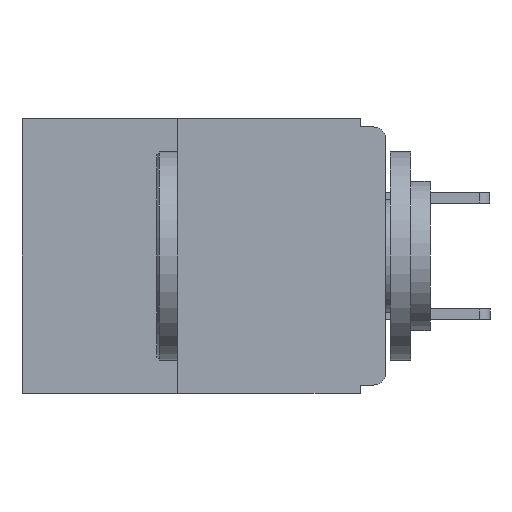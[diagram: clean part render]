
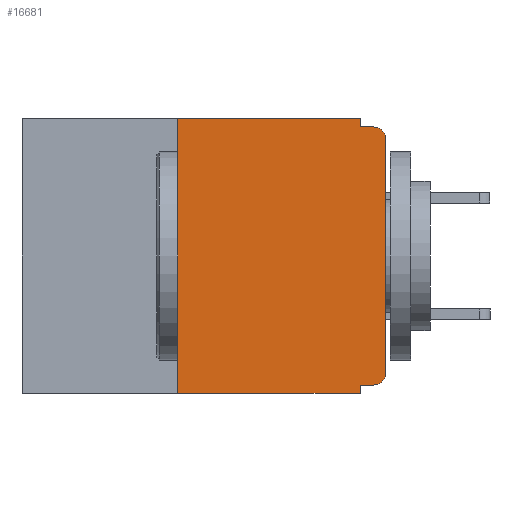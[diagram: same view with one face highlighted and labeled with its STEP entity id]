
A CAD part, left-side view. The second image highlights one B-rep face of the part: STEP entity #16681.
In plain terms, the highlighted planar face has unit normal (-1, 0, 0).
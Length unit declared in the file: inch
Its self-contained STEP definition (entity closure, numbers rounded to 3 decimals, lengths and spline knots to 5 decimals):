
#120 = CARTESIAN_POINT ( 'NONE',  ( 0., 0.031, 0. ) ) ;
#642 = ORIENTED_EDGE ( 'NONE', *, *, #11901, .F. ) ;
#661 = CIRCLE ( 'NONE', #12540, 0.015 ) ;
#827 = VERTEX_POINT ( 'NONE', #120 ) ;
#833 = LINE ( 'NONE', #2622, #10771 ) ;
#2117 = LINE ( 'NONE', #3980, #16971 ) ;
#2421 = ORIENTED_EDGE ( 'NONE', *, *, #15866, .T. ) ;
#2622 = CARTESIAN_POINT ( 'NONE',  ( 0., 0., -0.32 ) ) ;
#3060 = VECTOR ( 'NONE', #7362, 39.37008 ) ;
#3620 = CARTESIAN_POINT ( 'NONE',  ( 0., 0.437, -0.33 ) ) ;
#3735 = CARTESIAN_POINT ( 'NONE',  ( 0., 0.031, -0.32 ) ) ;
#3980 = CARTESIAN_POINT ( 'NONE',  ( 0., 0.031, -0.33 ) ) ;
#4224 = EDGE_CURVE ( 'NONE', #21188, #827, #18725, .T. ) ;
#5014 = VERTEX_POINT ( 'NONE', #8833 ) ;
#5261 = EDGE_LOOP ( 'NONE', ( #8554, #20725, #17062, #13027, #14784, #9329, #12256, #642, #23493, #2421 ) ) ;
#5452 = VERTEX_POINT ( 'NONE', #3735 ) ;
#5600 = CARTESIAN_POINT ( 'NONE',  ( 0., 0.437, 0. ) ) ;
#6415 = DIRECTION ( 'NONE',  ( 0., 1., 0. ) ) ;
#7362 = DIRECTION ( 'NONE',  ( 0., -1., 0. ) ) ;
#8055 = CARTESIAN_POINT ( 'NONE',  ( 0., 0.015, -0.025 ) ) ;
#8554 = ORIENTED_EDGE ( 'NONE', *, *, #17490, .T. ) ;
#8629 = DIRECTION ( 'NONE',  ( -1., 0., 0. ) ) ;
#8631 = DIRECTION ( 'NONE',  ( 0., 0., -1. ) ) ;
#8833 = CARTESIAN_POINT ( 'NONE',  ( 0., 0.015, -0.32 ) ) ;
#9329 = ORIENTED_EDGE ( 'NONE', *, *, #22744, .F. ) ;
#9636 = LINE ( 'NONE', #21296, #18838 ) ;
#9851 = CARTESIAN_POINT ( 'NONE',  ( 0., 0., 0. ) ) ;
#9900 = DIRECTION ( 'NONE',  ( 0., 0., -1. ) ) ;
#10041 = CARTESIAN_POINT ( 'NONE',  ( 0., 0.031, -0.33 ) ) ;
#10771 = VECTOR ( 'NONE', #6415, 39.37008 ) ;
#10929 = VERTEX_POINT ( 'NONE', #10041 ) ;
#11167 = DIRECTION ( 'NONE',  ( 0., 0., -1. ) ) ;
#11192 = CARTESIAN_POINT ( 'NONE',  ( 0., 0.25, -0.33 ) ) ;
#11901 = EDGE_CURVE ( 'NONE', #5452, #10929, #2117, .T. ) ;
#12256 = ORIENTED_EDGE ( 'NONE', *, *, #14221, .T. ) ;
#12506 = CIRCLE ( 'NONE', #22842, 0.015 ) ;
#12531 = VECTOR ( 'NONE', #8631, 39.37008 ) ;
#12540 = AXIS2_PLACEMENT_3D ( 'NONE', #19636, #8629, #21514 ) ;
#12827 = VECTOR ( 'NONE', #15337, 39.37008 ) ;
#12979 = DIRECTION ( 'NONE',  ( 0., 0., 1. ) ) ;
#13014 = VERTEX_POINT ( 'NONE', #16906 ) ;
#13027 = ORIENTED_EDGE ( 'NONE', *, *, #17704, .F. ) ;
#13408 = DIRECTION ( 'NONE',  ( 0., -1., 0. ) ) ;
#13815 = VECTOR ( 'NONE', #12979, 39.37008 ) ;
#13829 = CARTESIAN_POINT ( 'NONE',  ( 0., 0.031, -0.01 ) ) ;
#13869 = VECTOR ( 'NONE', #13408, 39.37008 ) ;
#13952 = CARTESIAN_POINT ( 'NONE',  ( 0., 0.437, 0. ) ) ;
#14221 = EDGE_CURVE ( 'NONE', #20856, #10929, #17867, .T. ) ;
#14546 = VERTEX_POINT ( 'NONE', #23185 ) ;
#14784 = ORIENTED_EDGE ( 'NONE', *, *, #4224, .F. ) ;
#15095 = DIRECTION ( 'NONE',  ( 0., 0., -1. ) ) ;
#15127 = VERTEX_POINT ( 'NONE', #13829 ) ;
#15337 = DIRECTION ( 'NONE',  ( 0., 0., 1. ) ) ;
#15866 = EDGE_CURVE ( 'NONE', #5014, #13014, #661, .T. ) ;
#16170 = CARTESIAN_POINT ( 'NONE',  ( 0., 0.25, -0.33 ) ) ;
#16210 = CARTESIAN_POINT ( 'NONE',  ( 0., 0.015, -0.01 ) ) ;
#16681 = ADVANCED_FACE ( 'NONE', ( #17778 ), #20344, .F. ) ;
#16906 = CARTESIAN_POINT ( 'NONE',  ( 0., 0., -0.305 ) ) ;
#16971 = VECTOR ( 'NONE', #15095, 39.37008 ) ;
#17062 = ORIENTED_EDGE ( 'NONE', *, *, #18919, .F. ) ;
#17447 = LINE ( 'NONE', #17825, #12531 ) ;
#17490 = EDGE_CURVE ( 'NONE', #13014, #14546, #17739, .T. ) ;
#17704 = EDGE_CURVE ( 'NONE', #827, #15127, #17447, .T. ) ;
#17739 = LINE ( 'NONE', #9851, #12827 ) ;
#17778 = FACE_OUTER_BOUND ( 'NONE', #5261, .T. ) ;
#17825 = CARTESIAN_POINT ( 'NONE',  ( 0., 0.031, 0. ) ) ;
#17867 = LINE ( 'NONE', #3620, #3060 ) ;
#18149 = EDGE_CURVE ( 'NONE', #14546, #23050, #12506, .T. ) ;
#18251 = EDGE_CURVE ( 'NONE', #5014, #5452, #833, .T. ) ;
#18725 = LINE ( 'NONE', #13952, #13869 ) ;
#18838 = VECTOR ( 'NONE', #23076, 39.37008 ) ;
#18919 = EDGE_CURVE ( 'NONE', #15127, #23050, #9636, .T. ) ;
#19636 = CARTESIAN_POINT ( 'NONE',  ( 0., 0.015, -0.305 ) ) ;
#20344 = PLANE ( 'NONE',  #22666 ) ;
#20725 = ORIENTED_EDGE ( 'NONE', *, *, #18149, .T. ) ;
#20856 = VERTEX_POINT ( 'NONE', #16170 ) ;
#20940 = DIRECTION ( 'NONE',  ( -1., 0., 0. ) ) ;
#21188 = VERTEX_POINT ( 'NONE', #23116 ) ;
#21296 = CARTESIAN_POINT ( 'NONE',  ( 0., 0., -0.01 ) ) ;
#21514 = DIRECTION ( 'NONE',  ( 0., 0., -1. ) ) ;
#22178 = DIRECTION ( 'NONE',  ( 1., 0., 0. ) ) ;
#22666 = AXIS2_PLACEMENT_3D ( 'NONE', #5600, #22178, #11167 ) ;
#22744 = EDGE_CURVE ( 'NONE', #20856, #21188, #22947, .T. ) ;
#22842 = AXIS2_PLACEMENT_3D ( 'NONE', #8055, #20940, #9900 ) ;
#22947 = LINE ( 'NONE', #11192, #13815 ) ;
#23050 = VERTEX_POINT ( 'NONE', #16210 ) ;
#23076 = DIRECTION ( 'NONE',  ( 0., -1., 0. ) ) ;
#23116 = CARTESIAN_POINT ( 'NONE',  ( 0., 0.25, 0. ) ) ;
#23185 = CARTESIAN_POINT ( 'NONE',  ( 0., 0., -0.025 ) ) ;
#23493 = ORIENTED_EDGE ( 'NONE', *, *, #18251, .F. ) ;
